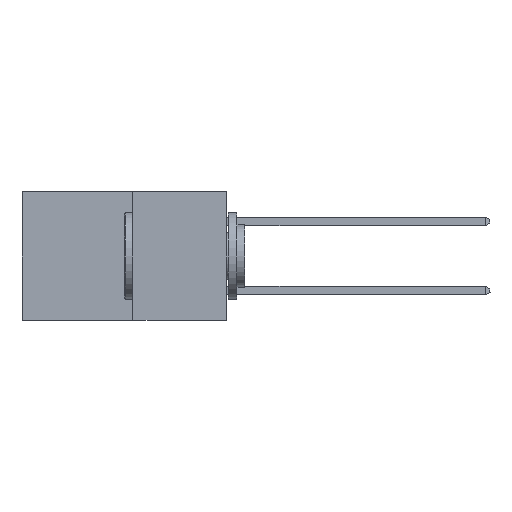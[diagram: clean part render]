
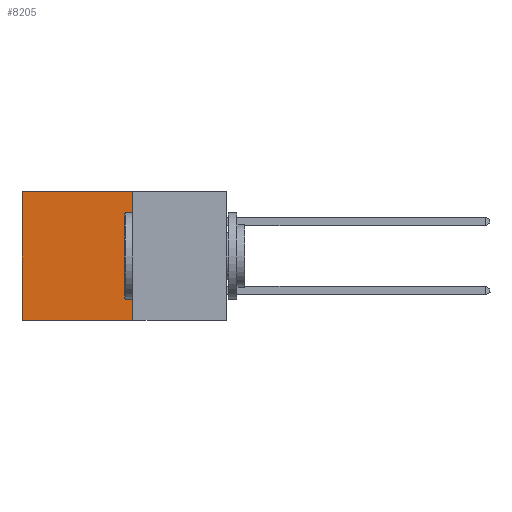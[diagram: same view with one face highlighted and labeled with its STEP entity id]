
A CAD part, left-side view. The second image highlights one B-rep face of the part: STEP entity #8205.
In plain terms, the highlighted planar face has unit normal (-1, 0, 0).
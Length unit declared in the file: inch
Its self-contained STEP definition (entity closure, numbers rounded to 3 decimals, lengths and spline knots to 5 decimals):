
#663 = VECTOR ( 'NONE', #24077, 39.37008 ) ;
#959 = CARTESIAN_POINT ( 'NONE',  ( 0.277, 0.27, 0. ) ) ;
#2275 = ORIENTED_EDGE ( 'NONE', *, *, #4278, .F. ) ;
#2713 = VECTOR ( 'NONE', #7800, 39.37008 ) ;
#2976 = DIRECTION ( 'NONE',  ( 1., 0., 0. ) ) ;
#4167 = ORIENTED_EDGE ( 'NONE', *, *, #15034, .T. ) ;
#4278 = EDGE_CURVE ( 'NONE', #21627, #30985, #16631, .T. ) ;
#4387 = EDGE_CURVE ( 'NONE', #24313, #21627, #7110, .T. ) ;
#5301 = CARTESIAN_POINT ( 'NONE',  ( 0.277, 0.27, -0.37 ) ) ;
#6323 = VERTEX_POINT ( 'NONE', #13169 ) ;
#6611 = CARTESIAN_POINT ( 'NONE',  ( 0.277, 0.59, -0.37 ) ) ;
#6867 = ORIENTED_EDGE ( 'NONE', *, *, #9643, .T. ) ;
#7036 = FACE_OUTER_BOUND ( 'NONE', #31143, .T. ) ;
#7110 = LINE ( 'NONE', #24292, #663 ) ;
#7800 = DIRECTION ( 'NONE',  ( 0., 0., -1. ) ) ;
#8205 = ADVANCED_FACE ( 'NONE', ( #7036 ), #19872, .F. ) ;
#9195 = LINE ( 'NONE', #17330, #2713 ) ;
#9643 = EDGE_CURVE ( 'NONE', #24313, #6323, #11914, .T. ) ;
#10184 = VECTOR ( 'NONE', #16829, 39.37008 ) ;
#11914 = LINE ( 'NONE', #959, #30571 ) ;
#13169 = CARTESIAN_POINT ( 'NONE',  ( 0.277, 0.59, 0. ) ) ;
#13396 = CARTESIAN_POINT ( 'NONE',  ( 0.277, 0.27, -0.37 ) ) ;
#15034 = EDGE_CURVE ( 'NONE', #6323, #30985, #9195, .T. ) ;
#16631 = LINE ( 'NONE', #21522, #10184 ) ;
#16829 = DIRECTION ( 'NONE',  ( 0., 1., 0. ) ) ;
#17330 = CARTESIAN_POINT ( 'NONE',  ( 0.277, 0.59, -0.37 ) ) ;
#19872 = PLANE ( 'NONE',  #22971 ) ;
#19969 = DIRECTION ( 'NONE',  ( 0., 0., -1. ) ) ;
#20355 = CARTESIAN_POINT ( 'NONE',  ( 0.277, 0.27, 0. ) ) ;
#21522 = CARTESIAN_POINT ( 'NONE',  ( 0.277, 0.27, -0.37 ) ) ;
#21627 = VERTEX_POINT ( 'NONE', #13396 ) ;
#22862 = DIRECTION ( 'NONE',  ( 0., 1., 0. ) ) ;
#22971 = AXIS2_PLACEMENT_3D ( 'NONE', #5301, #2976, #19969 ) ;
#24077 = DIRECTION ( 'NONE',  ( 0., 0., -1. ) ) ;
#24292 = CARTESIAN_POINT ( 'NONE',  ( 0.277, 0.27, -0.37 ) ) ;
#24313 = VERTEX_POINT ( 'NONE', #20355 ) ;
#28062 = ORIENTED_EDGE ( 'NONE', *, *, #4387, .F. ) ;
#30571 = VECTOR ( 'NONE', #22862, 39.37008 ) ;
#30985 = VERTEX_POINT ( 'NONE', #6611 ) ;
#31143 = EDGE_LOOP ( 'NONE', ( #4167, #2275, #28062, #6867 ) ) ;
